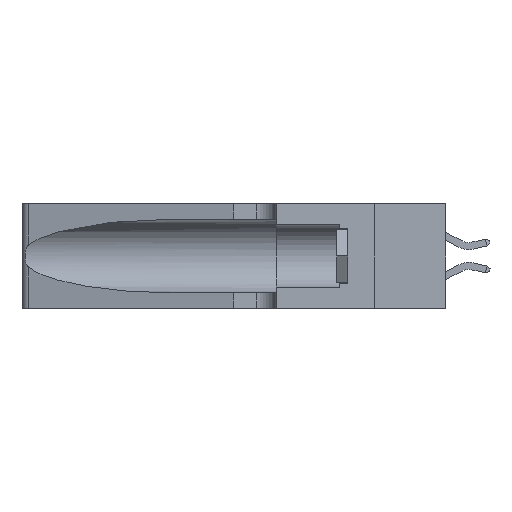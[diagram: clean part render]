
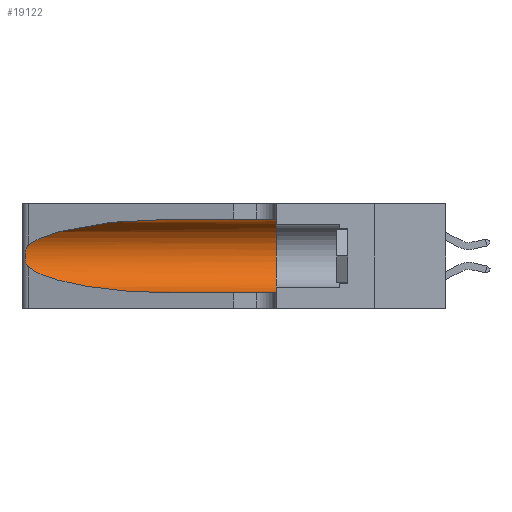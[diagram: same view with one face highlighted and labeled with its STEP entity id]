
A CAD part, left-side view. The second image highlights one B-rep face of the part: STEP entity #19122.
In plain terms, the highlighted cylindrical face has radius 3.308 mm (diameter 6.617 mm), a partial arc.
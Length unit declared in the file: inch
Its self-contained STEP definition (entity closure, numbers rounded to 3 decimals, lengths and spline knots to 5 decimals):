
#242 = CARTESIAN_POINT ( 'NONE',  ( 0.1305, 1.61858, 0.05475 ) ) ;
#676 = CARTESIAN_POINT ( 'NONE',  ( 0.2373, 1.15595, 0.28018 ) ) ;
#2406 = LINE ( 'NONE', #35873, #4311 ) ;
#2464 = DIRECTION ( 'NONE',  ( 0., 1., 0. ) ) ;
#2951 = CARTESIAN_POINT ( 'NONE',  ( 0.25854, 1.2359, 0.20912 ) ) ;
#3173 =( BOUNDED_CURVE ( )  B_SPLINE_CURVE ( 3, ( #19149, #31390, #25124, #7174 ),
 .UNSPECIFIED., .F., .T. ) 
 B_SPLINE_CURVE_WITH_KNOTS ( ( 4, 4 ),
 ( 3.44316, 4.71239 ),
 .UNSPECIFIED. ) 
 CURVE ( )  GEOMETRIC_REPRESENTATION_ITEM ( )  RATIONAL_B_SPLINE_CURVE ( ( 1., 0.87, 0.87, 1. ) ) 
 REPRESENTATION_ITEM ( '' )  );
#3575 = CARTESIAN_POINT ( 'NONE',  ( 0.25555, 1.22993, 0.14849 ) ) ;
#3706 = CARTESIAN_POINT ( 'NONE',  ( 0.1305, 0.35, 0.05475 ) ) ;
#4162 = ORIENTED_EDGE ( 'NONE', *, *, #25334, .T. ) ;
#4311 = VECTOR ( 'NONE', #16034, 39.37008 ) ;
#6003 = CARTESIAN_POINT ( 'NONE',  ( 0.26018, 1.23835, 0.19895 ) ) ;
#7174 = CARTESIAN_POINT ( 'NONE',  ( 0.1305, 0.72297, 0.05475 ) ) ;
#9992 = CARTESIAN_POINT ( 'NONE',  ( 0.1305, 1.61858, 0.185 ) ) ;
#10655 = CARTESIAN_POINT ( 'NONE',  ( 0.25487, 1.22718, 0.14631 ) ) ;
#10880 = CARTESIAN_POINT ( 'NONE',  ( 0.1305, 0.35, 0.185 ) ) ;
#11707 = ORIENTED_EDGE ( 'NONE', *, *, #22940, .T. ) ;
#11860 = CARTESIAN_POINT ( 'NONE',  ( 0.25639, 1.23184, 0.21858 ) ) ;
#12530 = CARTESIAN_POINT ( 'NONE',  ( 0.1305, 0.72297, 0.31525 ) ) ;
#12579 = CYLINDRICAL_SURFACE ( 'NONE', #32051, 0.13025 ) ;
#13588 = ORIENTED_EDGE ( 'NONE', *, *, #30177, .T. ) ;
#14669 = VERTEX_POINT ( 'NONE', #10655 ) ;
#14935 = AXIS2_PLACEMENT_3D ( 'NONE', #10880, #2464, #38506 ) ;
#15018 = DIRECTION ( 'NONE',  ( 0., -1., 0. ) ) ;
#15424 = CARTESIAN_POINT ( 'NONE',  ( 0.25487, 1.22718, 0.22369 ) ) ;
#16034 = DIRECTION ( 'NONE',  ( 0., -1., 0. ) ) ;
#16234 = CARTESIAN_POINT ( 'NONE',  ( 0.1305, 0.72297, 0.05475 ) ) ;
#17363 = ORIENTED_EDGE ( 'NONE', *, *, #36647, .F. ) ;
#18489 = CARTESIAN_POINT ( 'NONE',  ( 0.18966, 0.96281, 0.31525 ) ) ;
#18575 = CARTESIAN_POINT ( 'NONE',  ( 0.25856, 1.23593, 0.16098 ) ) ;
#18718 = CARTESIAN_POINT ( 'NONE',  ( 0.26075, 1.23896, 0.178 ) ) ;
#18847 =( BOUNDED_CURVE ( )  B_SPLINE_CURVE ( 3, ( #12530, #18489, #676, #15424 ),
 .UNSPECIFIED., .F., .T. ) 
 B_SPLINE_CURVE_WITH_KNOTS ( ( 4, 4 ),
 ( 1.5708, 2.84003 ),
 .UNSPECIFIED. ) 
 CURVE ( )  GEOMETRIC_REPRESENTATION_ITEM ( )  RATIONAL_B_SPLINE_CURVE ( ( 1., 0.87, 0.87, 1. ) ) 
 REPRESENTATION_ITEM ( '' )  );
#19122 = ADVANCED_FACE ( 'NONE', ( #23051 ), #12579, .F. ) ;
#19149 = CARTESIAN_POINT ( 'NONE',  ( 0.25487, 1.22718, 0.14631 ) ) ;
#21140 = CARTESIAN_POINT ( 'NONE',  ( 0.26075, 1.23896, 0.19203 ) ) ;
#22072 = CARTESIAN_POINT ( 'NONE',  ( 0.26017, 1.23833, 0.17102 ) ) ;
#22089 = DIRECTION ( 'NONE',  ( 0., -1., 0. ) ) ;
#22656 = VERTEX_POINT ( 'NONE', #34867 ) ;
#22940 = EDGE_CURVE ( 'NONE', #22656, #25018, #18847, .T. ) ;
#23051 = FACE_OUTER_BOUND ( 'NONE', #27053, .T. ) ;
#23932 = DIRECTION ( 'NONE',  ( 0., 0., -1. ) ) ;
#24055 = CARTESIAN_POINT ( 'NONE',  ( 0.25487, 1.22718, 0.22369 ) ) ;
#24894 = B_SPLINE_CURVE_WITH_KNOTS ( 'NONE', 3,
 ( #24055, #30426, #11860, #36165, #2951, #6003, #21140, #18718, #22072, #18575, #27646, #30819, #3575, #28038 ),
 .UNSPECIFIED., .F., .F.,
 ( 4, 2, 2, 2, 2, 2, 4 ),
 ( 0., 0.00027, 0.00053, 0.00107, 0.0016, 0.00187, 0.00214 ),
 .UNSPECIFIED. ) ;
#25018 = VERTEX_POINT ( 'NONE', #37415 ) ;
#25124 = CARTESIAN_POINT ( 'NONE',  ( 0.18966, 0.96281, 0.05475 ) ) ;
#25334 = EDGE_CURVE ( 'NONE', #34164, #32937, #29701, .T. ) ;
#27053 = EDGE_LOOP ( 'NONE', ( #11707, #32574, #13588, #4162, #17363, #38786 ) ) ;
#27646 = CARTESIAN_POINT ( 'NONE',  ( 0.25789, 1.23486, 0.15765 ) ) ;
#28038 = CARTESIAN_POINT ( 'NONE',  ( 0.25487, 1.22718, 0.14631 ) ) ;
#28899 = EDGE_CURVE ( 'NONE', #22656, #29953, #2406, .T. ) ;
#29701 = LINE ( 'NONE', #242, #33019 ) ;
#29953 = VERTEX_POINT ( 'NONE', #39012 ) ;
#30177 = EDGE_CURVE ( 'NONE', #14669, #34164, #3173, .T. ) ;
#30426 = CARTESIAN_POINT ( 'NONE',  ( 0.25555, 1.22994, 0.2215 ) ) ;
#30819 = CARTESIAN_POINT ( 'NONE',  ( 0.25639, 1.23186, 0.15144 ) ) ;
#31390 = CARTESIAN_POINT ( 'NONE',  ( 0.2373, 1.15595, 0.08982 ) ) ;
#32051 = AXIS2_PLACEMENT_3D ( 'NONE', #9992, #22089, #23932 ) ;
#32574 = ORIENTED_EDGE ( 'NONE', *, *, #34599, .T. ) ;
#32937 = VERTEX_POINT ( 'NONE', #3706 ) ;
#33019 = VECTOR ( 'NONE', #15018, 39.37008 ) ;
#33103 = CIRCLE ( 'NONE', #14935, 0.13025 ) ;
#34164 = VERTEX_POINT ( 'NONE', #16234 ) ;
#34599 = EDGE_CURVE ( 'NONE', #25018, #14669, #24894, .T. ) ;
#34867 = CARTESIAN_POINT ( 'NONE',  ( 0.1305, 0.72297, 0.31525 ) ) ;
#35873 = CARTESIAN_POINT ( 'NONE',  ( 0.1305, 1.61858, 0.31525 ) ) ;
#36165 = CARTESIAN_POINT ( 'NONE',  ( 0.25787, 1.23484, 0.2124 ) ) ;
#36647 = EDGE_CURVE ( 'NONE', #29953, #32937, #33103, .T. ) ;
#37415 = CARTESIAN_POINT ( 'NONE',  ( 0.25487, 1.22718, 0.22369 ) ) ;
#38506 = DIRECTION ( 'NONE',  ( 0., 0., 1. ) ) ;
#38786 = ORIENTED_EDGE ( 'NONE', *, *, #28899, .F. ) ;
#39012 = CARTESIAN_POINT ( 'NONE',  ( 0.1305, 0.35, 0.31525 ) ) ;
